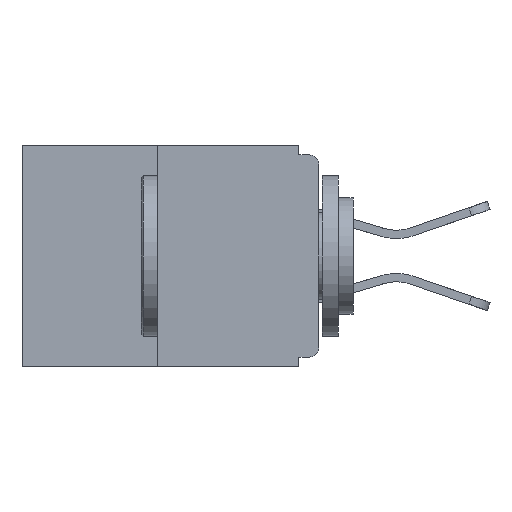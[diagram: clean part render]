
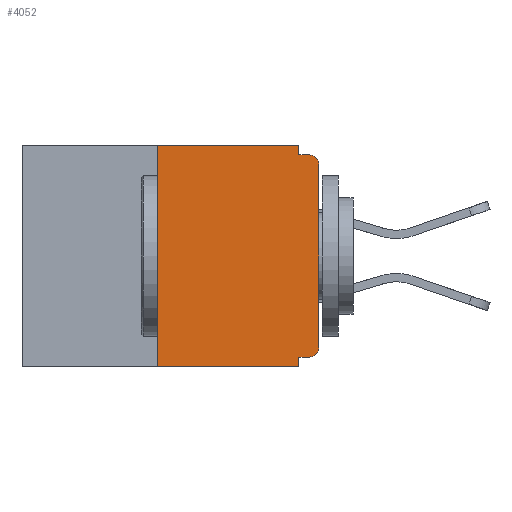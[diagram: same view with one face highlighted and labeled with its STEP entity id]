
A CAD part, left-side view. The second image highlights one B-rep face of the part: STEP entity #4052.
In plain terms, the highlighted planar face has unit normal (-1, 0, 0).
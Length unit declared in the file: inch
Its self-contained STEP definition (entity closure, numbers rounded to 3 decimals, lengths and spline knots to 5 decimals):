
#225 = VECTOR ( 'NONE', #1521, 39.37008 ) ;
#596 = ORIENTED_EDGE ( 'NONE', *, *, #10176, .F. ) ;
#1521 = DIRECTION ( 'NONE',  ( 0., -1., 0. ) ) ;
#1979 = CIRCLE ( 'NONE', #14587, 0.015 ) ;
#2417 = LINE ( 'NONE', #6989, #20054 ) ;
#2979 = VERTEX_POINT ( 'NONE', #16510 ) ;
#2996 = VERTEX_POINT ( 'NONE', #15062 ) ;
#3013 = ORIENTED_EDGE ( 'NONE', *, *, #8343, .T. ) ;
#3017 = ORIENTED_EDGE ( 'NONE', *, *, #12671, .F. ) ;
#3177 = CARTESIAN_POINT ( 'NONE',  ( 0., 0., -0.328 ) ) ;
#3659 = CARTESIAN_POINT ( 'NONE',  ( 0., 0.015, -0.313 ) ) ;
#3849 = EDGE_CURVE ( 'NONE', #3851, #11609, #20271, .T. ) ;
#3851 = VERTEX_POINT ( 'NONE', #14170 ) ;
#4052 = ADVANCED_FACE ( 'NONE', ( #4111 ), #11596, .F. ) ;
#4111 = FACE_OUTER_BOUND ( 'NONE', #15855, .T. ) ;
#4876 = CARTESIAN_POINT ( 'NONE',  ( 0., 0.46, 0. ) ) ;
#5292 = DIRECTION ( 'NONE',  ( 0., 0., -1. ) ) ;
#5588 = LINE ( 'NONE', #14973, #10476 ) ;
#5902 = LINE ( 'NONE', #17353, #10545 ) ;
#6854 = CARTESIAN_POINT ( 'NONE',  ( 0., 0.46, 0. ) ) ;
#6989 = CARTESIAN_POINT ( 'NONE',  ( 0., 0.031, -0.343 ) ) ;
#7653 = CARTESIAN_POINT ( 'NONE',  ( 0., 0.015, -0.328 ) ) ;
#7678 = EDGE_CURVE ( 'NONE', #18514, #2996, #9587, .T. ) ;
#8331 = VERTEX_POINT ( 'NONE', #18783 ) ;
#8343 = EDGE_CURVE ( 'NONE', #2996, #9426, #1979, .T. ) ;
#8601 = CARTESIAN_POINT ( 'NONE',  ( 0., 0., 0. ) ) ;
#8608 = AXIS2_PLACEMENT_3D ( 'NONE', #6854, #14658, #5292 ) ;
#8612 = VERTEX_POINT ( 'NONE', #14181 ) ;
#8644 = EDGE_CURVE ( 'NONE', #12871, #3851, #5902, .T. ) ;
#8684 = DIRECTION ( 'NONE',  ( 0., 0., -1. ) ) ;
#8752 = LINE ( 'NONE', #18384, #20260 ) ;
#8857 = CARTESIAN_POINT ( 'NONE',  ( 0., 0.015, -0.03 ) ) ;
#8919 = VECTOR ( 'NONE', #12644, 39.37008 ) ;
#9276 = ORIENTED_EDGE ( 'NONE', *, *, #12181, .T. ) ;
#9426 = VERTEX_POINT ( 'NONE', #11346 ) ;
#9587 = LINE ( 'NONE', #8601, #14250 ) ;
#10176 = EDGE_CURVE ( 'NONE', #8331, #9426, #5588, .T. ) ;
#10244 = EDGE_CURVE ( 'NONE', #11609, #8331, #8752, .T. ) ;
#10386 = ORIENTED_EDGE ( 'NONE', *, *, #17065, .T. ) ;
#10476 = VECTOR ( 'NONE', #18129, 39.37008 ) ;
#10532 = ORIENTED_EDGE ( 'NONE', *, *, #10244, .F. ) ;
#10540 = VECTOR ( 'NONE', #16419, 39.37008 ) ;
#10545 = VECTOR ( 'NONE', #14321, 39.37008 ) ;
#10569 = DIRECTION ( 'NONE',  ( -1., 0., 0. ) ) ;
#10579 = DIRECTION ( 'NONE',  ( 0., 0., -1. ) ) ;
#11346 = CARTESIAN_POINT ( 'NONE',  ( 0., 0.015, -0.015 ) ) ;
#11596 = PLANE ( 'NONE',  #8608 ) ;
#11609 = VERTEX_POINT ( 'NONE', #17177 ) ;
#12030 = DIRECTION ( 'NONE',  ( 0., 0., -1. ) ) ;
#12181 = EDGE_CURVE ( 'NONE', #15045, #18514, #17788, .T. ) ;
#12644 = DIRECTION ( 'NONE',  ( 0., 1., 0. ) ) ;
#12671 = EDGE_CURVE ( 'NONE', #15045, #2979, #19702, .T. ) ;
#12761 = LINE ( 'NONE', #14971, #10540 ) ;
#12871 = VERTEX_POINT ( 'NONE', #15096 ) ;
#14170 = CARTESIAN_POINT ( 'NONE',  ( 0., 0.25, 0. ) ) ;
#14181 = CARTESIAN_POINT ( 'NONE',  ( 0., 0.031, -0.343 ) ) ;
#14250 = VECTOR ( 'NONE', #19560, 39.37008 ) ;
#14321 = DIRECTION ( 'NONE',  ( 0., 0., 1. ) ) ;
#14587 = AXIS2_PLACEMENT_3D ( 'NONE', #8857, #10569, #12030 ) ;
#14658 = DIRECTION ( 'NONE',  ( 1., 0., 0. ) ) ;
#14820 = DIRECTION ( 'NONE',  ( -1., 0., 0. ) ) ;
#14971 = CARTESIAN_POINT ( 'NONE',  ( 0., 0.46, -0.343 ) ) ;
#14973 = CARTESIAN_POINT ( 'NONE',  ( 0., 0., -0.015 ) ) ;
#15045 = VERTEX_POINT ( 'NONE', #7653 ) ;
#15062 = CARTESIAN_POINT ( 'NONE',  ( 0., 0., -0.03 ) ) ;
#15096 = CARTESIAN_POINT ( 'NONE',  ( 0., 0.25, -0.343 ) ) ;
#15115 = ORIENTED_EDGE ( 'NONE', *, *, #7678, .T. ) ;
#15490 = EDGE_CURVE ( 'NONE', #2979, #8612, #2417, .T. ) ;
#15855 = EDGE_LOOP ( 'NONE', ( #19028, #19125, #10386, #16776, #3017, #9276, #15115, #3013, #596, #10532 ) ) ;
#16419 = DIRECTION ( 'NONE',  ( 0., -1., 0. ) ) ;
#16510 = CARTESIAN_POINT ( 'NONE',  ( 0., 0.031, -0.328 ) ) ;
#16776 = ORIENTED_EDGE ( 'NONE', *, *, #15490, .F. ) ;
#17065 = EDGE_CURVE ( 'NONE', #12871, #8612, #12761, .T. ) ;
#17177 = CARTESIAN_POINT ( 'NONE',  ( 0., 0.031, 0. ) ) ;
#17353 = CARTESIAN_POINT ( 'NONE',  ( 0., 0.25, 0. ) ) ;
#17788 = CIRCLE ( 'NONE', #18313, 0.015 ) ;
#18129 = DIRECTION ( 'NONE',  ( 0., -1., 0. ) ) ;
#18313 = AXIS2_PLACEMENT_3D ( 'NONE', #3659, #14820, #19464 ) ;
#18384 = CARTESIAN_POINT ( 'NONE',  ( 0., 0.031, 0. ) ) ;
#18514 = VERTEX_POINT ( 'NONE', #19274 ) ;
#18783 = CARTESIAN_POINT ( 'NONE',  ( 0., 0.031, -0.015 ) ) ;
#19028 = ORIENTED_EDGE ( 'NONE', *, *, #3849, .F. ) ;
#19125 = ORIENTED_EDGE ( 'NONE', *, *, #8644, .F. ) ;
#19274 = CARTESIAN_POINT ( 'NONE',  ( 0., 0., -0.313 ) ) ;
#19464 = DIRECTION ( 'NONE',  ( 0., 0., -1. ) ) ;
#19560 = DIRECTION ( 'NONE',  ( 0., 0., 1. ) ) ;
#19702 = LINE ( 'NONE', #3177, #8919 ) ;
#20054 = VECTOR ( 'NONE', #8684, 39.37008 ) ;
#20260 = VECTOR ( 'NONE', #10579, 39.37008 ) ;
#20271 = LINE ( 'NONE', #4876, #225 ) ;
